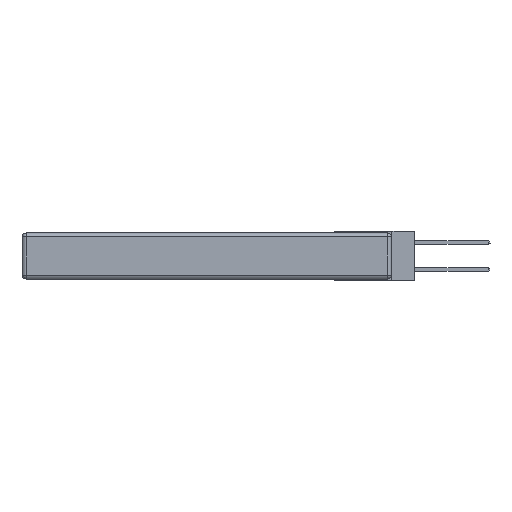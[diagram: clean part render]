
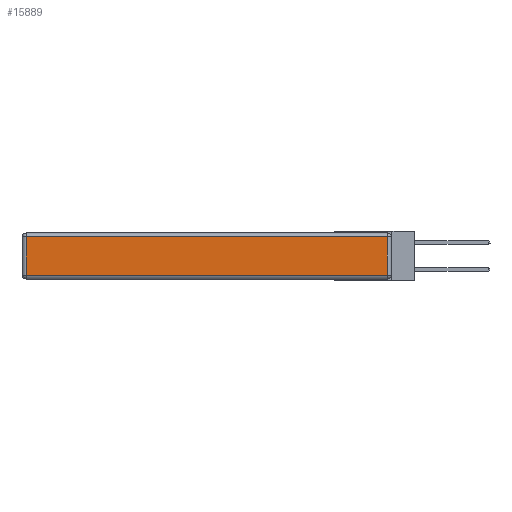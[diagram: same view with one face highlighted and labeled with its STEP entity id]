
A CAD part, left-side view. The second image highlights one B-rep face of the part: STEP entity #15889.
In plain terms, the highlighted planar face has unit normal (-1, 0, 0).
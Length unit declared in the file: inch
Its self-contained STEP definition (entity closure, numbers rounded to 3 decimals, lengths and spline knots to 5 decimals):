
#593 = LINE ( 'NONE', #5577, #12328 ) ;
#1447 = AXIS2_PLACEMENT_3D ( 'NONE', #12109, #6347, #6291 ) ;
#1517 = CARTESIAN_POINT ( 'NONE',  ( 0., 2.75, -0.03 ) ) ;
#2914 = VECTOR ( 'NONE', #13871, 39.37008 ) ;
#3756 = CARTESIAN_POINT ( 'NONE',  ( 0., 2.72, -0.03 ) ) ;
#4236 = DIRECTION ( 'NONE',  ( 0., 0., 1. ) ) ;
#4282 = CARTESIAN_POINT ( 'NONE',  ( 0., 2.72, -0.313 ) ) ;
#4482 = LINE ( 'NONE', #16760, #2914 ) ;
#5528 = DIRECTION ( 'NONE',  ( 0., 1., 0. ) ) ;
#5577 = CARTESIAN_POINT ( 'NONE',  ( 0., 0.03, -0.343 ) ) ;
#6062 = VERTEX_POINT ( 'NONE', #14459 ) ;
#6184 = EDGE_CURVE ( 'NONE', #17378, #8732, #7395, .T. ) ;
#6291 = DIRECTION ( 'NONE',  ( 0., 0., 1. ) ) ;
#6305 = FACE_OUTER_BOUND ( 'NONE', #13709, .T. ) ;
#6347 = DIRECTION ( 'NONE',  ( -1., 0., 0. ) ) ;
#6464 = DIRECTION ( 'NONE',  ( 0., -1., 0. ) ) ;
#6850 = ORIENTED_EDGE ( 'NONE', *, *, #16012, .T. ) ;
#7197 = EDGE_CURVE ( 'NONE', #8732, #6062, #593, .T. ) ;
#7395 = LINE ( 'NONE', #14662, #12620 ) ;
#8732 = VERTEX_POINT ( 'NONE', #12003 ) ;
#9709 = LINE ( 'NONE', #1517, #18295 ) ;
#10778 = ORIENTED_EDGE ( 'NONE', *, *, #7197, .T. ) ;
#12003 = CARTESIAN_POINT ( 'NONE',  ( 0., 0.03, -0.313 ) ) ;
#12109 = CARTESIAN_POINT ( 'NONE',  ( 0., 0., -0.343 ) ) ;
#12328 = VECTOR ( 'NONE', #4236, 39.37008 ) ;
#12620 = VECTOR ( 'NONE', #6464, 39.37008 ) ;
#12926 = ORIENTED_EDGE ( 'NONE', *, *, #16957, .T. ) ;
#13674 = VERTEX_POINT ( 'NONE', #3756 ) ;
#13709 = EDGE_LOOP ( 'NONE', ( #16552, #10778, #12926, #6850 ) ) ;
#13871 = DIRECTION ( 'NONE',  ( 0., 0., -1. ) ) ;
#14459 = CARTESIAN_POINT ( 'NONE',  ( 0., 0.03, -0.03 ) ) ;
#14662 = CARTESIAN_POINT ( 'NONE',  ( 0., 0., -0.313 ) ) ;
#15889 = ADVANCED_FACE ( 'NONE', ( #6305 ), #17860, .T. ) ;
#16012 = EDGE_CURVE ( 'NONE', #13674, #17378, #4482, .T. ) ;
#16552 = ORIENTED_EDGE ( 'NONE', *, *, #6184, .T. ) ;
#16760 = CARTESIAN_POINT ( 'NONE',  ( 0., 2.72, -0.343 ) ) ;
#16957 = EDGE_CURVE ( 'NONE', #6062, #13674, #9709, .T. ) ;
#17378 = VERTEX_POINT ( 'NONE', #4282 ) ;
#17860 = PLANE ( 'NONE',  #1447 ) ;
#18295 = VECTOR ( 'NONE', #5528, 39.37008 ) ;
